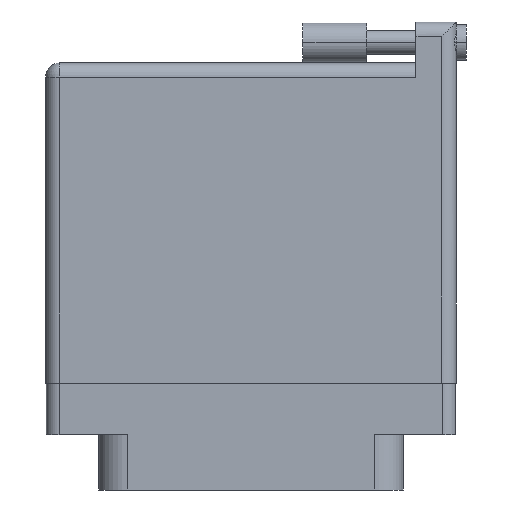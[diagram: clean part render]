
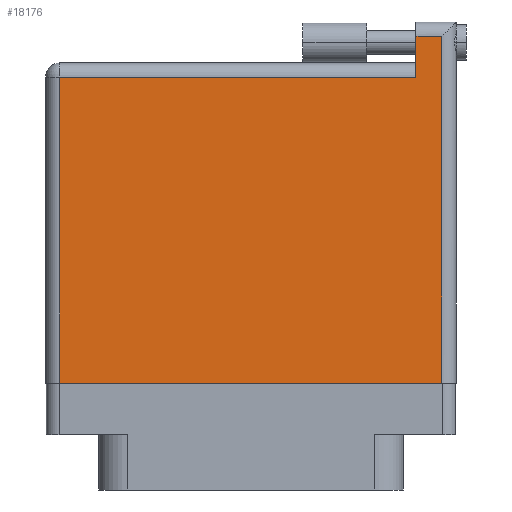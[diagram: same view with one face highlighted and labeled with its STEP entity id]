
A CAD part, front view. The second image highlights one B-rep face of the part: STEP entity #18176.
In plain terms, the highlighted face is planar.
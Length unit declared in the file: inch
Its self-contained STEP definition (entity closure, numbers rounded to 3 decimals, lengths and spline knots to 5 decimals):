
#1056 = VERTEX_POINT ( 'NONE', #5524 ) ;
#1088 = CARTESIAN_POINT ( 'NONE',  ( -0.934, 1.396, 0.4495 ) ) ;
#1389 = VERTEX_POINT ( 'NONE', #1912 ) ;
#1912 = CARTESIAN_POINT ( 'NONE',  ( 0.934, 1.596, 0.4495 ) ) ;
#1987 = VERTEX_POINT ( 'NONE', #1088 ) ;
#2403 = CARTESIAN_POINT ( 'NONE',  ( 0.807, 1.666, 0.4495 ) ) ;
#3080 = CARTESIAN_POINT ( 'NONE',  ( -1.004, 1.466, 0.4495 ) ) ;
#3530 = EDGE_CURVE ( 'NONE', #5317, #1987, #22324, .T. ) ;
#4015 = AXIS2_PLACEMENT_3D ( 'NONE', #3080, #33548, #28080 ) ;
#5059 = ORIENTED_EDGE ( 'NONE', *, *, #28233, .T. ) ;
#5317 = VERTEX_POINT ( 'NONE', #9443 ) ;
#5524 = CARTESIAN_POINT ( 'NONE',  ( -0.934, -0.1, 0.4495 ) ) ;
#5814 = VECTOR ( 'NONE', #24599, 39.37008 ) ;
#6947 = ORIENTED_EDGE ( 'NONE', *, *, #32272, .T. ) ;
#7392 = LINE ( 'NONE', #30566, #13837 ) ;
#9443 = CARTESIAN_POINT ( 'NONE',  ( 0.807, 1.396, 0.4495 ) ) ;
#9551 = CARTESIAN_POINT ( 'NONE',  ( -1.004, 1.396, 0.4495 ) ) ;
#9751 = CARTESIAN_POINT ( 'NONE',  ( -1.004, -0.1, 0.4495 ) ) ;
#11419 = EDGE_CURVE ( 'NONE', #1389, #15770, #31364, .T. ) ;
#11483 = VECTOR ( 'NONE', #23028, 39.37008 ) ;
#11635 = ORIENTED_EDGE ( 'NONE', *, *, #3530, .T. ) ;
#13501 = EDGE_LOOP ( 'NONE', ( #15418, #6947, #17247, #17669, #11635, #5059 ) ) ;
#13837 = VECTOR ( 'NONE', #16782, 39.37008 ) ;
#13903 = DIRECTION ( 'NONE',  ( 0., -1., 0. ) ) ;
#14020 = VERTEX_POINT ( 'NONE', #17245 ) ;
#14941 = VECTOR ( 'NONE', #25755, 39.37008 ) ;
#15418 = ORIENTED_EDGE ( 'NONE', *, *, #33718, .T. ) ;
#15770 = VERTEX_POINT ( 'NONE', #30954 ) ;
#16782 = DIRECTION ( 'NONE',  ( 0., 1., 0. ) ) ;
#16861 = VECTOR ( 'NONE', #34415, 39.37008 ) ;
#17245 = CARTESIAN_POINT ( 'NONE',  ( 0.934, -0.1, 0.4495 ) ) ;
#17247 = ORIENTED_EDGE ( 'NONE', *, *, #11419, .T. ) ;
#17669 = ORIENTED_EDGE ( 'NONE', *, *, #19410, .T. ) ;
#18176 = ADVANCED_FACE ( 'NONE', ( #31440 ), #27732, .F. ) ;
#19410 = EDGE_CURVE ( 'NONE', #15770, #5317, #28740, .T. ) ;
#22076 = LINE ( 'NONE', #9751, #16861 ) ;
#22324 = LINE ( 'NONE', #9551, #14941 ) ;
#22900 = CARTESIAN_POINT ( 'NONE',  ( -1.004, 1.596, 0.4495 ) ) ;
#23028 = DIRECTION ( 'NONE',  ( -1., 0., 0. ) ) ;
#24599 = DIRECTION ( 'NONE',  ( 0., -1., 0. ) ) ;
#24994 = VECTOR ( 'NONE', #13903, 39.37008 ) ;
#25755 = DIRECTION ( 'NONE',  ( -1., 0., 0. ) ) ;
#27708 = CARTESIAN_POINT ( 'NONE',  ( -0.934, -0.1, 0.4495 ) ) ;
#27732 = PLANE ( 'NONE',  #4015 ) ;
#28080 = DIRECTION ( 'NONE',  ( -1., 0., 0. ) ) ;
#28233 = EDGE_CURVE ( 'NONE', #1987, #1056, #34530, .T. ) ;
#28740 = LINE ( 'NONE', #2403, #5814 ) ;
#30566 = CARTESIAN_POINT ( 'NONE',  ( 0.934, 1.666, 0.4495 ) ) ;
#30954 = CARTESIAN_POINT ( 'NONE',  ( 0.807, 1.596, 0.4495 ) ) ;
#31364 = LINE ( 'NONE', #22900, #11483 ) ;
#31440 = FACE_OUTER_BOUND ( 'NONE', #13501, .T. ) ;
#32272 = EDGE_CURVE ( 'NONE', #14020, #1389, #7392, .T. ) ;
#33548 = DIRECTION ( 'NONE',  ( 0., 0., -1. ) ) ;
#33718 = EDGE_CURVE ( 'NONE', #1056, #14020, #22076, .T. ) ;
#34415 = DIRECTION ( 'NONE',  ( 1., 0., 0. ) ) ;
#34530 = LINE ( 'NONE', #27708, #24994 ) ;
